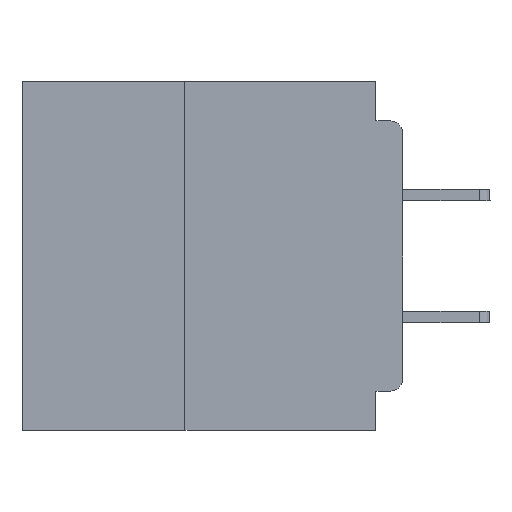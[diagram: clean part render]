
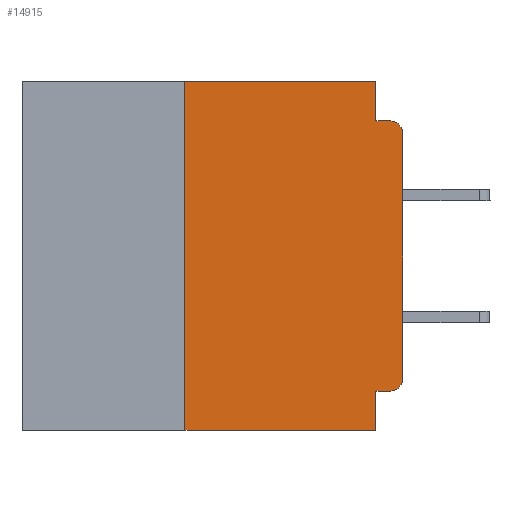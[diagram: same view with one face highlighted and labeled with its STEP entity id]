
A CAD part, left-side view. The second image highlights one B-rep face of the part: STEP entity #14915.
In plain terms, the highlighted planar face has unit normal (-1, 0, 0).
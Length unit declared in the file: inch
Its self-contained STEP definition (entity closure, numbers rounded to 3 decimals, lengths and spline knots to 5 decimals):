
#9 = CARTESIAN_POINT ( 'NONE',  ( 0., 0., 0. ) ) ;
#745 = CARTESIAN_POINT ( 'NONE',  ( 0., 0.437, -0.4 ) ) ;
#927 = DIRECTION ( 'NONE',  ( 1., 0., 0. ) ) ;
#1098 = LINE ( 'NONE', #49506, #39543 ) ;
#2771 = DIRECTION ( 'NONE',  ( 0., 0., -1. ) ) ;
#4164 = CARTESIAN_POINT ( 'NONE',  ( 0., 0., -0.045 ) ) ;
#4272 = VERTEX_POINT ( 'NONE', #52675 ) ;
#5201 = DIRECTION ( 'NONE',  ( 0., 1., 0. ) ) ;
#5291 = DIRECTION ( 'NONE',  ( 0., 0., 1. ) ) ;
#6141 = VERTEX_POINT ( 'NONE', #20891 ) ;
#7136 = EDGE_CURVE ( 'NONE', #10100, #4272, #14896, .T. ) ;
#9352 = VERTEX_POINT ( 'NONE', #52372 ) ;
#9474 = CARTESIAN_POINT ( 'NONE',  ( 0., 0.015, -0.34 ) ) ;
#10100 = VERTEX_POINT ( 'NONE', #22180 ) ;
#11530 = CARTESIAN_POINT ( 'NONE',  ( 0., 0.015, -0.045 ) ) ;
#11938 = DIRECTION ( 'NONE',  ( 0., 0., 1. ) ) ;
#12785 = CARTESIAN_POINT ( 'NONE',  ( 0., 0.25, -0.4 ) ) ;
#13539 = VERTEX_POINT ( 'NONE', #20459 ) ;
#13774 = ORIENTED_EDGE ( 'NONE', *, *, #35076, .T. ) ;
#13911 = ORIENTED_EDGE ( 'NONE', *, *, #64672, .T. ) ;
#14751 = DIRECTION ( 'NONE',  ( 0., 0., -1. ) ) ;
#14896 = LINE ( 'NONE', #65102, #54748 ) ;
#14915 = ADVANCED_FACE ( 'NONE', ( #32578 ), #32293, .F. ) ;
#15494 = CARTESIAN_POINT ( 'NONE',  ( 0., 0.437, 0. ) ) ;
#15502 = ORIENTED_EDGE ( 'NONE', *, *, #23061, .F. ) ;
#16744 = ORIENTED_EDGE ( 'NONE', *, *, #29442, .F. ) ;
#17089 = ORIENTED_EDGE ( 'NONE', *, *, #36291, .F. ) ;
#17253 = VECTOR ( 'NONE', #63119, 39.37008 ) ;
#18418 = DIRECTION ( 'NONE',  ( 0., 0., -1. ) ) ;
#18434 = ORIENTED_EDGE ( 'NONE', *, *, #35205, .F. ) ;
#18713 = ORIENTED_EDGE ( 'NONE', *, *, #40156, .T. ) ;
#19674 = VECTOR ( 'NONE', #18418, 39.37008 ) ;
#19889 = ORIENTED_EDGE ( 'NONE', *, *, #7136, .F. ) ;
#20139 = ORIENTED_EDGE ( 'NONE', *, *, #65473, .F. ) ;
#20459 = CARTESIAN_POINT ( 'NONE',  ( 0., 0., -0.34 ) ) ;
#20817 = DIRECTION ( 'NONE',  ( 0., -1., 0. ) ) ;
#20891 = CARTESIAN_POINT ( 'NONE',  ( 0., 0.25, 0. ) ) ;
#21004 = CIRCLE ( 'NONE', #52970, 0.015 ) ;
#21330 = ORIENTED_EDGE ( 'NONE', *, *, #64681, .T. ) ;
#21849 = VERTEX_POINT ( 'NONE', #35749 ) ;
#22134 = LINE ( 'NONE', #4164, #44799 ) ;
#22180 = CARTESIAN_POINT ( 'NONE',  ( 0., 0.031, -0.355 ) ) ;
#23061 = EDGE_CURVE ( 'NONE', #37375, #38873, #22134, .T. ) ;
#25121 = DIRECTION ( 'NONE',  ( -1., 0., 0. ) ) ;
#26292 = VECTOR ( 'NONE', #5291, 39.37008 ) ;
#26813 = LINE ( 'NONE', #15494, #52720 ) ;
#26873 = VERTEX_POINT ( 'NONE', #28761 ) ;
#28649 = CARTESIAN_POINT ( 'NONE',  ( 0., 0.031, 0. ) ) ;
#28761 = CARTESIAN_POINT ( 'NONE',  ( 0., 0.031, 0. ) ) ;
#29442 = EDGE_CURVE ( 'NONE', #26873, #37375, #33451, .T. ) ;
#32293 = PLANE ( 'NONE',  #60831 ) ;
#32578 = FACE_OUTER_BOUND ( 'NONE', #46981, .T. ) ;
#33451 = LINE ( 'NONE', #28649, #19674 ) ;
#35076 = EDGE_CURVE ( 'NONE', #13539, #21849, #53823, .T. ) ;
#35205 = EDGE_CURVE ( 'NONE', #50172, #6141, #57858, .T. ) ;
#35749 = CARTESIAN_POINT ( 'NONE',  ( 0., 0., -0.06 ) ) ;
#36291 = EDGE_CURVE ( 'NONE', #6141, #26873, #26813, .T. ) ;
#37375 = VERTEX_POINT ( 'NONE', #50419 ) ;
#37523 = DIRECTION ( 'NONE',  ( 0., 0., -1. ) ) ;
#38873 = VERTEX_POINT ( 'NONE', #11530 ) ;
#39543 = VECTOR ( 'NONE', #5201, 39.37008 ) ;
#40156 = EDGE_CURVE ( 'NONE', #50172, #4272, #44879, .T. ) ;
#44799 = VECTOR ( 'NONE', #61480, 39.37008 ) ;
#44879 = LINE ( 'NONE', #745, #17253 ) ;
#45921 = DIRECTION ( 'NONE',  ( -1., 0., 0. ) ) ;
#46981 = EDGE_LOOP ( 'NONE', ( #13774, #13911, #15502, #16744, #17089, #18434, #18713, #19889, #20139, #21330 ) ) ;
#49506 = CARTESIAN_POINT ( 'NONE',  ( 0., 0., -0.355 ) ) ;
#50172 = VERTEX_POINT ( 'NONE', #12785 ) ;
#50419 = CARTESIAN_POINT ( 'NONE',  ( 0., 0.031, -0.045 ) ) ;
#52372 = CARTESIAN_POINT ( 'NONE',  ( 0., 0.015, -0.355 ) ) ;
#52675 = CARTESIAN_POINT ( 'NONE',  ( 0., 0.031, -0.4 ) ) ;
#52720 = VECTOR ( 'NONE', #20817, 39.37008 ) ;
#52910 = CARTESIAN_POINT ( 'NONE',  ( 0., 0.437, 0. ) ) ;
#52970 = AXIS2_PLACEMENT_3D ( 'NONE', #56134, #25121, #61301 ) ;
#53823 = LINE ( 'NONE', #9, #26292 ) ;
#54748 = VECTOR ( 'NONE', #2771, 39.37008 ) ;
#56134 = CARTESIAN_POINT ( 'NONE',  ( 0., 0.015, -0.06 ) ) ;
#56256 = VECTOR ( 'NONE', #11938, 39.37008 ) ;
#57858 = LINE ( 'NONE', #63718, #56256 ) ;
#59914 = AXIS2_PLACEMENT_3D ( 'NONE', #9474, #45921, #14751 ) ;
#60702 = CIRCLE ( 'NONE', #59914, 0.015 ) ;
#60831 = AXIS2_PLACEMENT_3D ( 'NONE', #52910, #927, #37523 ) ;
#61301 = DIRECTION ( 'NONE',  ( 0., 0., -1. ) ) ;
#61480 = DIRECTION ( 'NONE',  ( 0., -1., 0. ) ) ;
#63119 = DIRECTION ( 'NONE',  ( 0., -1., 0. ) ) ;
#63718 = CARTESIAN_POINT ( 'NONE',  ( 0., 0.25, -0.4 ) ) ;
#64672 = EDGE_CURVE ( 'NONE', #21849, #38873, #21004, .T. ) ;
#64681 = EDGE_CURVE ( 'NONE', #9352, #13539, #60702, .T. ) ;
#65102 = CARTESIAN_POINT ( 'NONE',  ( 0., 0.031, -0.4 ) ) ;
#65473 = EDGE_CURVE ( 'NONE', #9352, #10100, #1098, .T. ) ;
